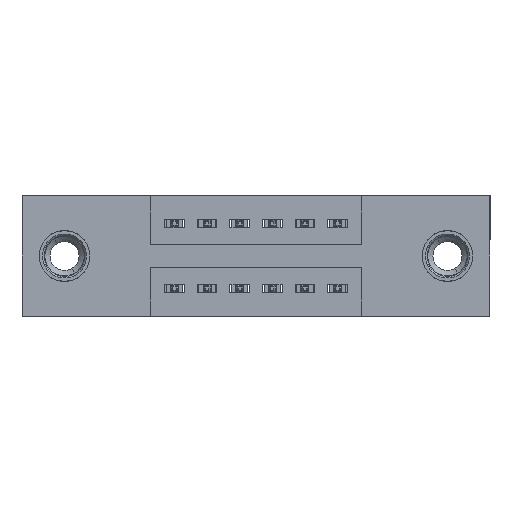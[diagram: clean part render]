
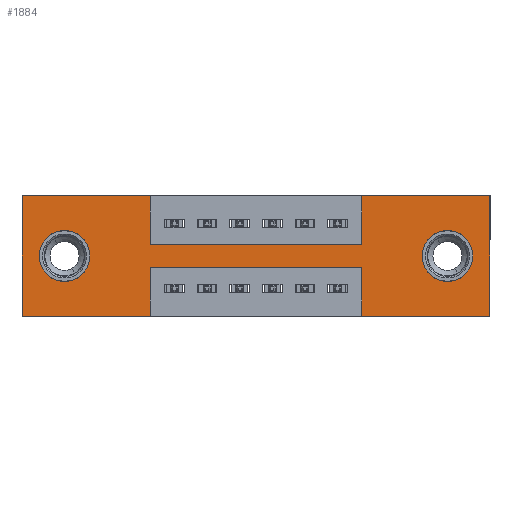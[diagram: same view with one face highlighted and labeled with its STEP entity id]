
A CAD part, front view. The second image highlights one B-rep face of the part: STEP entity #1884.
In plain terms, the highlighted planar face has unit normal (0, -1, 0).
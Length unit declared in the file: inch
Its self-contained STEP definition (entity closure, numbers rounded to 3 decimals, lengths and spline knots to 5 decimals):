
#99 = AXIS2_PLACEMENT_3D ( 'NONE', #4809, #6995, #2786 ) ;
#105 = CARTESIAN_POINT ( 'NONE',  ( 0.3925, 0., -0.37 ) ) ;
#214 = LINE ( 'NONE', #13705, #8466 ) ;
#275 = VECTOR ( 'NONE', #4099, 39.37008 ) ;
#553 = VERTEX_POINT ( 'NONE', #9692 ) ;
#568 = VECTOR ( 'NONE', #11345, 39.37008 ) ;
#855 = DIRECTION ( 'NONE',  ( 0., 0., 1. ) ) ;
#1009 = LINE ( 'NONE', #4174, #5881 ) ;
#1011 = VECTOR ( 'NONE', #8397, 39.37008 ) ;
#1186 = VERTEX_POINT ( 'NONE', #10025 ) ;
#1204 = AXIS2_PLACEMENT_3D ( 'NONE', #8956, #13433, #12036 ) ;
#1314 = LINE ( 'NONE', #13346, #2117 ) ;
#1411 = VECTOR ( 'NONE', #14131, 39.37008 ) ;
#1479 = ORIENTED_EDGE ( 'NONE', *, *, #5040, .F. ) ;
#1545 = ORIENTED_EDGE ( 'NONE', *, *, #5869, .F. ) ;
#1715 = EDGE_CURVE ( 'NONE', #553, #5164, #2970, .T. ) ;
#1848 = EDGE_CURVE ( 'NONE', #10355, #7248, #5618, .T. ) ;
#1853 = DIRECTION ( 'NONE',  ( 0., 0., 1. ) ) ;
#1884 = ADVANCED_FACE ( 'NONE', ( #12325, #11154, #10047 ), #13202, .T. ) ;
#2007 = CARTESIAN_POINT ( 'NONE',  ( 0.13, 0., -0.185 ) ) ;
#2076 = EDGE_CURVE ( 'NONE', #5930, #8922, #12752, .T. ) ;
#2117 = VECTOR ( 'NONE', #10269, 39.37008 ) ;
#2203 = CARTESIAN_POINT ( 'NONE',  ( 1.305, 0., -0.185 ) ) ;
#2308 = ORIENTED_EDGE ( 'NONE', *, *, #6264, .F. ) ;
#2577 = ORIENTED_EDGE ( 'NONE', *, *, #2990, .F. ) ;
#2786 = DIRECTION ( 'NONE',  ( 0., 0., -1. ) ) ;
#2795 = CARTESIAN_POINT ( 'NONE',  ( 0., 0., 0. ) ) ;
#2970 = CIRCLE ( 'NONE', #10410, 0.078 ) ;
#2990 = EDGE_CURVE ( 'NONE', #11510, #6220, #7096, .T. ) ;
#2999 = VERTEX_POINT ( 'NONE', #10576 ) ;
#3130 = EDGE_CURVE ( 'NONE', #8922, #5468, #1009, .T. ) ;
#3540 = VERTEX_POINT ( 'NONE', #4154 ) ;
#3637 = DIRECTION ( 'NONE',  ( 0., 0., 1. ) ) ;
#3655 = ORIENTED_EDGE ( 'NONE', *, *, #3130, .F. ) ;
#3693 = CARTESIAN_POINT ( 'NONE',  ( 0.3925, 0., 0. ) ) ;
#3699 = EDGE_LOOP ( 'NONE', ( #2308, #4639, #9253, #9837, #3655, #13792, #1479, #1545, #12332, #13870, #10254, #2577 ) ) ;
#4099 = DIRECTION ( 'NONE',  ( 1., 0., 0. ) ) ;
#4154 = CARTESIAN_POINT ( 'NONE',  ( 1.0425, 0., -0.15 ) ) ;
#4174 = CARTESIAN_POINT ( 'NONE',  ( 1.435, 0., 0. ) ) ;
#4287 = CARTESIAN_POINT ( 'NONE',  ( 0.3925, 0., -0.22 ) ) ;
#4308 = CIRCLE ( 'NONE', #99, 0.078 ) ;
#4639 = ORIENTED_EDGE ( 'NONE', *, *, #9138, .F. ) ;
#4809 = CARTESIAN_POINT ( 'NONE',  ( 1.305, 0., -0.185 ) ) ;
#5040 = EDGE_CURVE ( 'NONE', #3540, #5930, #11943, .T. ) ;
#5148 = EDGE_CURVE ( 'NONE', #5164, #553, #9605, .T. ) ;
#5151 = CARTESIAN_POINT ( 'NONE',  ( 1.0425, 0., -0.37 ) ) ;
#5164 = VERTEX_POINT ( 'NONE', #6444 ) ;
#5334 = CARTESIAN_POINT ( 'NONE',  ( 1.0425, 0., -0.37 ) ) ;
#5468 = VERTEX_POINT ( 'NONE', #10446 ) ;
#5497 = LINE ( 'NONE', #7850, #1411 ) ;
#5618 = CIRCLE ( 'NONE', #13080, 0.078 ) ;
#5735 = LINE ( 'NONE', #10015, #568 ) ;
#5869 = EDGE_CURVE ( 'NONE', #2999, #3540, #214, .T. ) ;
#5881 = VECTOR ( 'NONE', #8734, 39.37008 ) ;
#5885 = CARTESIAN_POINT ( 'NONE',  ( 0.3925, 0., -0.22 ) ) ;
#5930 = VERTEX_POINT ( 'NONE', #7208 ) ;
#5996 = CARTESIAN_POINT ( 'NONE',  ( 0., 0., -0.37 ) ) ;
#6197 = ORIENTED_EDGE ( 'NONE', *, *, #12231, .T. ) ;
#6220 = VERTEX_POINT ( 'NONE', #12523 ) ;
#6262 = ORIENTED_EDGE ( 'NONE', *, *, #5148, .T. ) ;
#6264 = EDGE_CURVE ( 'NONE', #7686, #11510, #5735, .T. ) ;
#6437 = EDGE_LOOP ( 'NONE', ( #11653, #6262 ) ) ;
#6444 = CARTESIAN_POINT ( 'NONE',  ( 0.13, 0., -0.263 ) ) ;
#6632 = LINE ( 'NONE', #12246, #10356 ) ;
#6971 = CARTESIAN_POINT ( 'NONE',  ( 1.305, 0., -0.107 ) ) ;
#6995 = DIRECTION ( 'NONE',  ( 0., 1., 0. ) ) ;
#7029 = DIRECTION ( 'NONE',  ( 0., 1., 0. ) ) ;
#7055 = VECTOR ( 'NONE', #8113, 39.37008 ) ;
#7096 = LINE ( 'NONE', #5996, #7055 ) ;
#7195 = CARTESIAN_POINT ( 'NONE',  ( 0., 0., 0. ) ) ;
#7208 = CARTESIAN_POINT ( 'NONE',  ( 1.0425, 0., 0. ) ) ;
#7248 = VERTEX_POINT ( 'NONE', #12320 ) ;
#7514 = VERTEX_POINT ( 'NONE', #5151 ) ;
#7562 = DIRECTION ( 'NONE',  ( 0., 0., 1. ) ) ;
#7686 = VERTEX_POINT ( 'NONE', #5885 ) ;
#7850 = CARTESIAN_POINT ( 'NONE',  ( 0., 0., -0.37 ) ) ;
#7885 = DIRECTION ( 'NONE',  ( 0., 1., 0. ) ) ;
#8113 = DIRECTION ( 'NONE',  ( -1., 0., 0. ) ) ;
#8397 = DIRECTION ( 'NONE',  ( 0., 0., -1. ) ) ;
#8466 = VECTOR ( 'NONE', #11017, 39.37008 ) ;
#8704 = DIRECTION ( 'NONE',  ( -1., 0., 0. ) ) ;
#8734 = DIRECTION ( 'NONE',  ( 0., 0., -1. ) ) ;
#8922 = VERTEX_POINT ( 'NONE', #11636 ) ;
#8956 = CARTESIAN_POINT ( 'NONE',  ( 0., 0., -0.37 ) ) ;
#9078 = VECTOR ( 'NONE', #7562, 39.37008 ) ;
#9138 = EDGE_CURVE ( 'NONE', #1186, #7686, #14253, .T. ) ;
#9253 = ORIENTED_EDGE ( 'NONE', *, *, #12803, .F. ) ;
#9605 = CIRCLE ( 'NONE', #12178, 0.078 ) ;
#9692 = CARTESIAN_POINT ( 'NONE',  ( 0.13, 0., -0.107 ) ) ;
#9837 = ORIENTED_EDGE ( 'NONE', *, *, #14235, .F. ) ;
#10015 = CARTESIAN_POINT ( 'NONE',  ( 0.3925, 0., -0.37 ) ) ;
#10025 = CARTESIAN_POINT ( 'NONE',  ( 1.0425, 0., -0.22 ) ) ;
#10047 = FACE_OUTER_BOUND ( 'NONE', #3699, .T. ) ;
#10254 = ORIENTED_EDGE ( 'NONE', *, *, #13211, .F. ) ;
#10269 = DIRECTION ( 'NONE',  ( 0., 0., 1. ) ) ;
#10355 = VERTEX_POINT ( 'NONE', #6971 ) ;
#10356 = VECTOR ( 'NONE', #13568, 39.37008 ) ;
#10410 = AXIS2_PLACEMENT_3D ( 'NONE', #13605, #7029, #3637 ) ;
#10446 = CARTESIAN_POINT ( 'NONE',  ( 1.435, 0., -0.37 ) ) ;
#10558 = VECTOR ( 'NONE', #855, 39.37008 ) ;
#10576 = CARTESIAN_POINT ( 'NONE',  ( 0.3925, 0., -0.15 ) ) ;
#11017 = DIRECTION ( 'NONE',  ( 1., 0., 0. ) ) ;
#11154 = FACE_BOUND ( 'NONE', #6437, .T. ) ;
#11345 = DIRECTION ( 'NONE',  ( 0., 0., -1. ) ) ;
#11471 = ORIENTED_EDGE ( 'NONE', *, *, #1848, .T. ) ;
#11510 = VERTEX_POINT ( 'NONE', #105 ) ;
#11534 = EDGE_CURVE ( 'NONE', #11745, #2999, #12350, .T. ) ;
#11636 = CARTESIAN_POINT ( 'NONE',  ( 1.435, 0., 0. ) ) ;
#11653 = ORIENTED_EDGE ( 'NONE', *, *, #1715, .T. ) ;
#11745 = VERTEX_POINT ( 'NONE', #3693 ) ;
#11907 = VECTOR ( 'NONE', #8704, 39.37008 ) ;
#11943 = LINE ( 'NONE', #14271, #10558 ) ;
#12036 = DIRECTION ( 'NONE',  ( 0., 0., -1. ) ) ;
#12137 = EDGE_CURVE ( 'NONE', #13661, #11745, #6632, .T. ) ;
#12178 = AXIS2_PLACEMENT_3D ( 'NONE', #2007, #12935, #1853 ) ;
#12231 = EDGE_CURVE ( 'NONE', #7248, #10355, #4308, .T. ) ;
#12246 = CARTESIAN_POINT ( 'NONE',  ( 0., 0., 0. ) ) ;
#12258 = DIRECTION ( 'NONE',  ( 0., 0., -1. ) ) ;
#12320 = CARTESIAN_POINT ( 'NONE',  ( 1.305, 0., -0.263 ) ) ;
#12325 = FACE_BOUND ( 'NONE', #12514, .T. ) ;
#12332 = ORIENTED_EDGE ( 'NONE', *, *, #11534, .F. ) ;
#12350 = LINE ( 'NONE', #12841, #1011 ) ;
#12514 = EDGE_LOOP ( 'NONE', ( #11471, #6197 ) ) ;
#12523 = CARTESIAN_POINT ( 'NONE',  ( 0., 0., -0.37 ) ) ;
#12752 = LINE ( 'NONE', #2795, #275 ) ;
#12803 = EDGE_CURVE ( 'NONE', #7514, #1186, #13161, .T. ) ;
#12841 = CARTESIAN_POINT ( 'NONE',  ( 0.3925, 0., 0. ) ) ;
#12935 = DIRECTION ( 'NONE',  ( 0., 1., 0. ) ) ;
#13080 = AXIS2_PLACEMENT_3D ( 'NONE', #2203, #7885, #12258 ) ;
#13161 = LINE ( 'NONE', #5334, #9078 ) ;
#13202 = PLANE ( 'NONE',  #1204 ) ;
#13211 = EDGE_CURVE ( 'NONE', #6220, #13661, #1314, .T. ) ;
#13346 = CARTESIAN_POINT ( 'NONE',  ( 0., 0., 0. ) ) ;
#13433 = DIRECTION ( 'NONE',  ( 0., -1., 0. ) ) ;
#13568 = DIRECTION ( 'NONE',  ( 1., 0., 0. ) ) ;
#13605 = CARTESIAN_POINT ( 'NONE',  ( 0.13, 0., -0.185 ) ) ;
#13661 = VERTEX_POINT ( 'NONE', #7195 ) ;
#13705 = CARTESIAN_POINT ( 'NONE',  ( 0.3925, 0., -0.15 ) ) ;
#13792 = ORIENTED_EDGE ( 'NONE', *, *, #2076, .F. ) ;
#13870 = ORIENTED_EDGE ( 'NONE', *, *, #12137, .F. ) ;
#14131 = DIRECTION ( 'NONE',  ( -1., 0., 0. ) ) ;
#14235 = EDGE_CURVE ( 'NONE', #5468, #7514, #5497, .T. ) ;
#14253 = LINE ( 'NONE', #4287, #11907 ) ;
#14271 = CARTESIAN_POINT ( 'NONE',  ( 1.0425, 0., 0. ) ) ;
